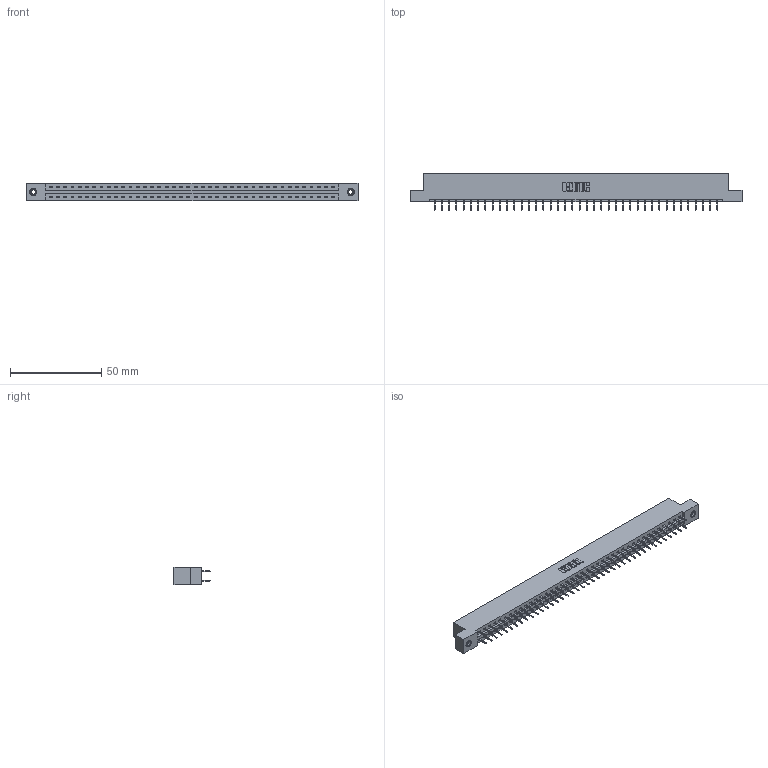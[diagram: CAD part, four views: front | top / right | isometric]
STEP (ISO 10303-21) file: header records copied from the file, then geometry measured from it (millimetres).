
FILE_DESCRIPTION (( 'STEP AP203' ), '1' );
FILE_NAME ('337-080-524-207.STEP', '2018-08-12T17:48:01', ( '' ), ( '' ), 'SwSTEP 2.0', 'SolidWorks 2016', '' );
FILE_SCHEMA (( 'CONFIG_CONTROL_DESIGN' ));
Length unit declared in the file: inch
Products named in the file (4): 345-250-001_345-250-005-103; 337-080-524-207; 337 Part_Flush Mounting Lugs - 0.156 Dia-TI; 345-292-001_345-293-124
Assembly tree (83 placements, depth 2):
  337-080-524-207
    337 Part_Flush Mounting Lugs - 0.156 Dia-TI
    345-292-001_345-293-124  x80
    345-250-001_345-250-005-103  x2
Bounding box: 181.51 x 19.69 x 9.4 mm (x, y, z)
Volume: 18967.6 mm3; surface area: 21084.5 mm2
Topology: 83 solids, 83 shells, 4814 faces, 13647 edges, 8770 vertices
Faces by surface type: plane 3622, cylinder 1176, cone 12, torus 4
Entity records: 32532 total; most frequent: CARTESIAN_POINT 5461, ORIENTED_EDGE 5390, DIRECTION 4681, EDGE_CURVE 2695, VECTOR 2551, LINE 2551, VERTEX_POINT 1788, AXIS2_PLACEMENT_3D 1065
